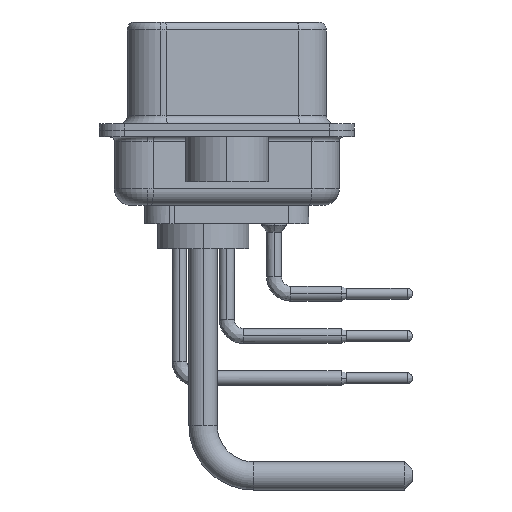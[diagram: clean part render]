
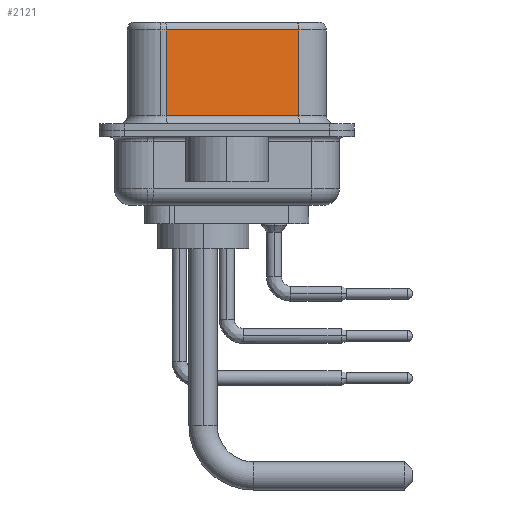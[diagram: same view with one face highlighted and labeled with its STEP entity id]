
A CAD part, left-side view. The second image highlights one B-rep face of the part: STEP entity #2121.
In plain terms, the highlighted planar face has unit normal (-0.985, -0.174, 0).
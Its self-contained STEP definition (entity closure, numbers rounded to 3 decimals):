
#276 = CARTESIAN_POINT ( 'NONE',  ( 3.73, 3.628, 6.02 ) ) ;
#1106 = LINE ( 'NONE', #14474, #25098 ) ;
#1752 = CARTESIAN_POINT ( 'NONE',  ( 5.132, -4.322, 6.52 ) ) ;
#2121 = ADVANCED_FACE ( 'NONE', ( #4522 ), #20694, .F. ) ;
#4522 = FACE_OUTER_BOUND ( 'NONE', #8511, .T. ) ;
#4727 = ORIENTED_EDGE ( 'NONE', *, *, #13912, .T. ) ;
#6546 = DIRECTION ( 'NONE',  ( 0., 0., -1. ) ) ;
#6789 = CARTESIAN_POINT ( 'NONE',  ( 5.132, -4.322, 6.02 ) ) ;
#7316 = DIRECTION ( 'NONE',  ( 0.174, -0.985, 0. ) ) ;
#8511 = EDGE_LOOP ( 'NONE', ( #33793, #4727, #18957, #18136 ) ) ;
#8984 = CARTESIAN_POINT ( 'NONE',  ( 3.73, 3.628, 6.52 ) ) ;
#9215 = VERTEX_POINT ( 'NONE', #21875 ) ;
#9386 = DIRECTION ( 'NONE',  ( -0.174, 0.985, 0. ) ) ;
#10138 = EDGE_CURVE ( 'NONE', #18016, #9215, #1106, .T. ) ;
#12200 = CARTESIAN_POINT ( 'NONE',  ( 5.132, -4.322, 6.02 ) ) ;
#12732 = VERTEX_POINT ( 'NONE', #276 ) ;
#13912 = EDGE_CURVE ( 'NONE', #18016, #12732, #21163, .T. ) ;
#14474 = CARTESIAN_POINT ( 'NONE',  ( 5.132, -4.322, 6.52 ) ) ;
#16352 = EDGE_CURVE ( 'NONE', #23359, #9215, #32827, .T. ) ;
#18016 = VERTEX_POINT ( 'NONE', #12200 ) ;
#18136 = ORIENTED_EDGE ( 'NONE', *, *, #16352, .T. ) ;
#18957 = ORIENTED_EDGE ( 'NONE', *, *, #22322, .T. ) ;
#19402 = VECTOR ( 'NONE', #6546, 1000. ) ;
#20694 = PLANE ( 'NONE',  #31577 ) ;
#20982 = VECTOR ( 'NONE', #9386, 1000. ) ;
#21163 = LINE ( 'NONE', #6789, #20982 ) ;
#21875 = CARTESIAN_POINT ( 'NONE',  ( 5.132, -4.322, 0.9 ) ) ;
#22322 = EDGE_CURVE ( 'NONE', #12732, #23359, #22538, .T. ) ;
#22538 = LINE ( 'NONE', #8984, #19402 ) ;
#23138 = CARTESIAN_POINT ( 'NONE',  ( 3.73, 3.628, 0.9 ) ) ;
#23359 = VERTEX_POINT ( 'NONE', #23138 ) ;
#25098 = VECTOR ( 'NONE', #30233, 1000. ) ;
#26033 = DIRECTION ( 'NONE',  ( -0.174, 0.985, 0. ) ) ;
#28641 = CARTESIAN_POINT ( 'NONE',  ( 5.132, -4.322, 0.9 ) ) ;
#30233 = DIRECTION ( 'NONE',  ( 0., 0., -1. ) ) ;
#31577 = AXIS2_PLACEMENT_3D ( 'NONE', #1752, #33986, #26033 ) ;
#32360 = VECTOR ( 'NONE', #7316, 1000. ) ;
#32827 = LINE ( 'NONE', #28641, #32360 ) ;
#33793 = ORIENTED_EDGE ( 'NONE', *, *, #10138, .F. ) ;
#33986 = DIRECTION ( 'NONE',  ( 0.985, 0.174, 0. ) ) ;
